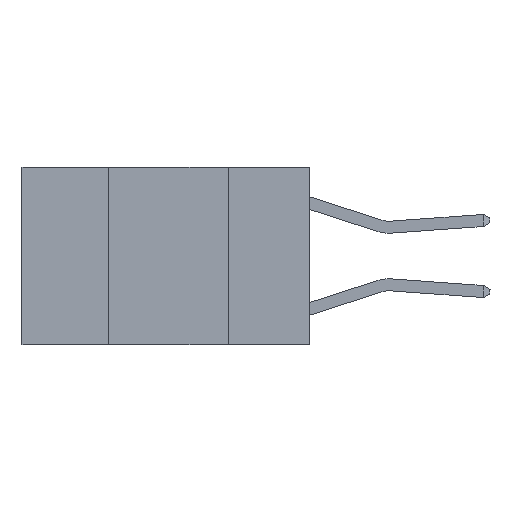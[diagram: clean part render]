
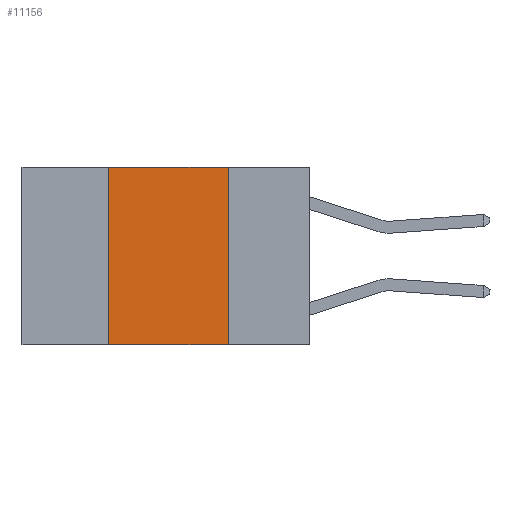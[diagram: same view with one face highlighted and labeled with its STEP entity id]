
A CAD part, left-side view. The second image highlights one B-rep face of the part: STEP entity #11156.
In plain terms, the highlighted planar face has unit normal (-1, 0, 0).
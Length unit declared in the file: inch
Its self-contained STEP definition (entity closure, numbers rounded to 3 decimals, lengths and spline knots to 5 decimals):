
#553 = DIRECTION ( 'NONE',  ( 1., 0., 0. ) ) ;
#1130 = DIRECTION ( 'NONE',  ( 0., -1., 0. ) ) ;
#1336 = VECTOR ( 'NONE', #9720, 39.37008 ) ;
#1395 = VECTOR ( 'NONE', #1130, 39.37008 ) ;
#1418 = CARTESIAN_POINT ( 'NONE',  ( 0., 0.17, 0. ) ) ;
#1970 = CARTESIAN_POINT ( 'NONE',  ( 0., 0.6, 0. ) ) ;
#2235 = FACE_OUTER_BOUND ( 'NONE', #8402, .T. ) ;
#2237 = CARTESIAN_POINT ( 'NONE',  ( 0., 0.17, -0.37 ) ) ;
#2509 = DIRECTION ( 'NONE',  ( 0., 0., -1. ) ) ;
#2734 = ORIENTED_EDGE ( 'NONE', *, *, #3591, .F. ) ;
#3073 = ORIENTED_EDGE ( 'NONE', *, *, #5054, .F. ) ;
#3245 = VERTEX_POINT ( 'NONE', #6235 ) ;
#3543 = CARTESIAN_POINT ( 'NONE',  ( 0., 0.42, 0. ) ) ;
#3591 = EDGE_CURVE ( 'NONE', #3245, #6491, #6457, .T. ) ;
#4732 = VERTEX_POINT ( 'NONE', #3543 ) ;
#4739 = VECTOR ( 'NONE', #11531, 39.37008 ) ;
#5054 = EDGE_CURVE ( 'NONE', #4732, #3245, #7578, .T. ) ;
#5716 = CARTESIAN_POINT ( 'NONE',  ( 0., 0.42, -0.37 ) ) ;
#5901 = ORIENTED_EDGE ( 'NONE', *, *, #7137, .F. ) ;
#6235 = CARTESIAN_POINT ( 'NONE',  ( 0., 0.17, 0. ) ) ;
#6457 = LINE ( 'NONE', #1418, #8946 ) ;
#6491 = VERTEX_POINT ( 'NONE', #2237 ) ;
#6911 = PLANE ( 'NONE',  #7420 ) ;
#6950 = CARTESIAN_POINT ( 'NONE',  ( 0., 0.6, 0. ) ) ;
#7065 = LINE ( 'NONE', #10726, #1395 ) ;
#7137 = EDGE_CURVE ( 'NONE', #8878, #4732, #9863, .T. ) ;
#7229 = ORIENTED_EDGE ( 'NONE', *, *, #10579, .T. ) ;
#7420 = AXIS2_PLACEMENT_3D ( 'NONE', #6950, #553, #8032 ) ;
#7578 = LINE ( 'NONE', #1970, #4739 ) ;
#8032 = DIRECTION ( 'NONE',  ( 0., 0., -1. ) ) ;
#8402 = EDGE_LOOP ( 'NONE', ( #2734, #3073, #5901, #7229 ) ) ;
#8632 = CARTESIAN_POINT ( 'NONE',  ( 0., 0.42, 0. ) ) ;
#8878 = VERTEX_POINT ( 'NONE', #5716 ) ;
#8946 = VECTOR ( 'NONE', #2509, 39.37008 ) ;
#9720 = DIRECTION ( 'NONE',  ( 0., 0., 1. ) ) ;
#9863 = LINE ( 'NONE', #8632, #1336 ) ;
#10579 = EDGE_CURVE ( 'NONE', #8878, #6491, #7065, .T. ) ;
#10726 = CARTESIAN_POINT ( 'NONE',  ( 0., 0.6, -0.37 ) ) ;
#11156 = ADVANCED_FACE ( 'NONE', ( #2235 ), #6911, .F. ) ;
#11531 = DIRECTION ( 'NONE',  ( 0., -1., 0. ) ) ;
